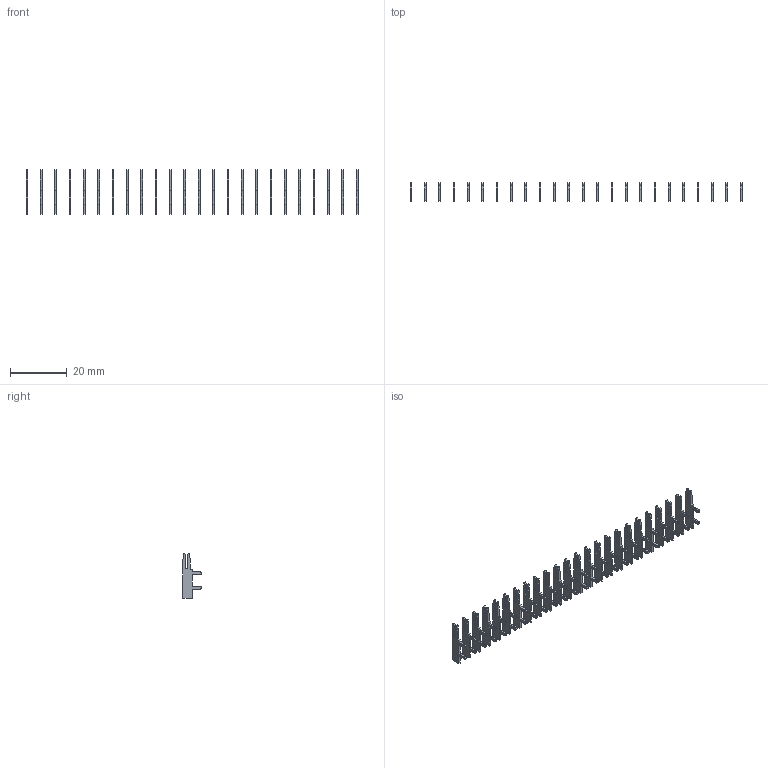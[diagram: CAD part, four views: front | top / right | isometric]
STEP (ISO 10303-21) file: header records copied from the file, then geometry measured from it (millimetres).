
FILE_DESCRIPTION (( 'STEP AP203' ), '1' );
FILE_NAME ('105-024-202-200.STEP', '2020-04-07T23:08:13', ( '' ), ( '' ), 'SwSTEP 2.0', 'SolidWorks 2016', '' );
FILE_SCHEMA (( 'CONFIG_CONTROL_DESIGN' ));
Length unit declared in the file: inch
Products named in the file (2): 105-024-202-200; 100-290-001_100-290-202
Assembly tree (24 placements, depth 2):
  105-024-202-200
    100-290-001_100-290-202  x24
Bounding box: 117.44 x 6.53 x 15.88 mm (x, y, z)
Volume: 762.5 mm3; surface area: 3391.2 mm2
Topology: 24 solids, 24 shells, 720 faces, 2016 edges, 1344 vertices
Faces by surface type: plane 552, cylinder 168
Entity records: 1898 total; most frequent: CARTESIAN_POINT 209, DIRECTION 208, ORIENTED_EDGE 168, EDGE_CURVE 84, AXIS2_PLACEMENT_3D 71, VECTOR 66, LINE 66, DATE_AND_TIME 58
